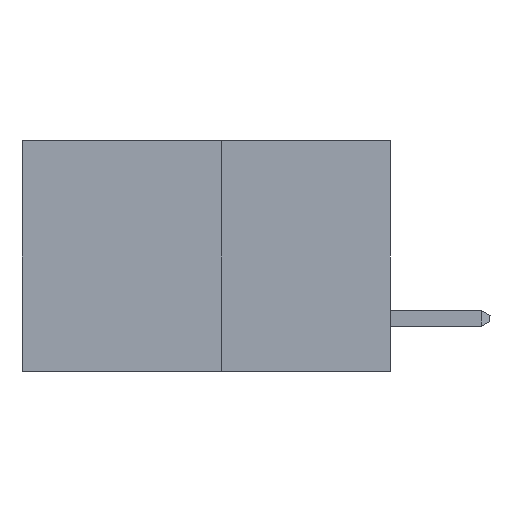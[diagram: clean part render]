
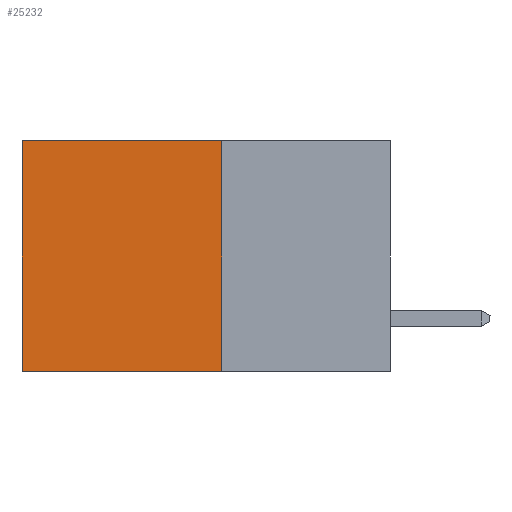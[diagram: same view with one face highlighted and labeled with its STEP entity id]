
A CAD part, left-side view. The second image highlights one B-rep face of the part: STEP entity #25232.
In plain terms, the highlighted planar face has unit normal (-1, 0, 0).
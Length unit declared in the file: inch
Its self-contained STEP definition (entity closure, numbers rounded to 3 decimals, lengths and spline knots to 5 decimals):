
#1886 = VECTOR ( 'NONE', #6678, 39.37008 ) ;
#4522 = CARTESIAN_POINT ( 'NONE',  ( 0.277, 0.59, -0.37 ) ) ;
#4531 = LINE ( 'NONE', #14834, #9527 ) ;
#5008 = LINE ( 'NONE', #5864, #21944 ) ;
#5500 = ORIENTED_EDGE ( 'NONE', *, *, #16599, .T. ) ;
#5864 = CARTESIAN_POINT ( 'NONE',  ( 0.277, 0.27, -0.37 ) ) ;
#6402 = DIRECTION ( 'NONE',  ( 0., 1., 0. ) ) ;
#6678 = DIRECTION ( 'NONE',  ( 0., 0., -1. ) ) ;
#7142 = CARTESIAN_POINT ( 'NONE',  ( 0.277, 0.27, 0. ) ) ;
#7764 = LINE ( 'NONE', #12536, #19030 ) ;
#7839 = ORIENTED_EDGE ( 'NONE', *, *, #18432, .F. ) ;
#8658 = VERTEX_POINT ( 'NONE', #7142 ) ;
#9085 = FACE_OUTER_BOUND ( 'NONE', #23866, .T. ) ;
#9527 = VECTOR ( 'NONE', #6402, 39.37008 ) ;
#11781 = PLANE ( 'NONE',  #16685 ) ;
#12536 = CARTESIAN_POINT ( 'NONE',  ( 0.277, 0.27, 0. ) ) ;
#13907 = DIRECTION ( 'NONE',  ( 0., 0., -1. ) ) ;
#14023 = VERTEX_POINT ( 'NONE', #26690 ) ;
#14295 = DIRECTION ( 'NONE',  ( 0., 0., -1. ) ) ;
#14834 = CARTESIAN_POINT ( 'NONE',  ( 0.277, 0.27, -0.37 ) ) ;
#15969 = VERTEX_POINT ( 'NONE', #17351 ) ;
#16307 = ORIENTED_EDGE ( 'NONE', *, *, #24793, .T. ) ;
#16599 = EDGE_CURVE ( 'NONE', #15969, #19303, #18844, .T. ) ;
#16685 = AXIS2_PLACEMENT_3D ( 'NONE', #20187, #26483, #13907 ) ;
#17351 = CARTESIAN_POINT ( 'NONE',  ( 0.277, 0.59, 0. ) ) ;
#18432 = EDGE_CURVE ( 'NONE', #14023, #19303, #4531, .T. ) ;
#18844 = LINE ( 'NONE', #4522, #1886 ) ;
#19030 = VECTOR ( 'NONE', #27211, 39.37008 ) ;
#19303 = VERTEX_POINT ( 'NONE', #22148 ) ;
#20187 = CARTESIAN_POINT ( 'NONE',  ( 0.277, 0.27, -0.37 ) ) ;
#21944 = VECTOR ( 'NONE', #14295, 39.37008 ) ;
#22148 = CARTESIAN_POINT ( 'NONE',  ( 0.277, 0.59, -0.37 ) ) ;
#23866 = EDGE_LOOP ( 'NONE', ( #5500, #7839, #25536, #16307 ) ) ;
#24793 = EDGE_CURVE ( 'NONE', #8658, #15969, #7764, .T. ) ;
#25232 = ADVANCED_FACE ( 'NONE', ( #9085 ), #11781, .F. ) ;
#25536 = ORIENTED_EDGE ( 'NONE', *, *, #26559, .F. ) ;
#26483 = DIRECTION ( 'NONE',  ( 1., 0., 0. ) ) ;
#26559 = EDGE_CURVE ( 'NONE', #8658, #14023, #5008, .T. ) ;
#26690 = CARTESIAN_POINT ( 'NONE',  ( 0.277, 0.27, -0.37 ) ) ;
#27211 = DIRECTION ( 'NONE',  ( 0., 1., 0. ) ) ;
